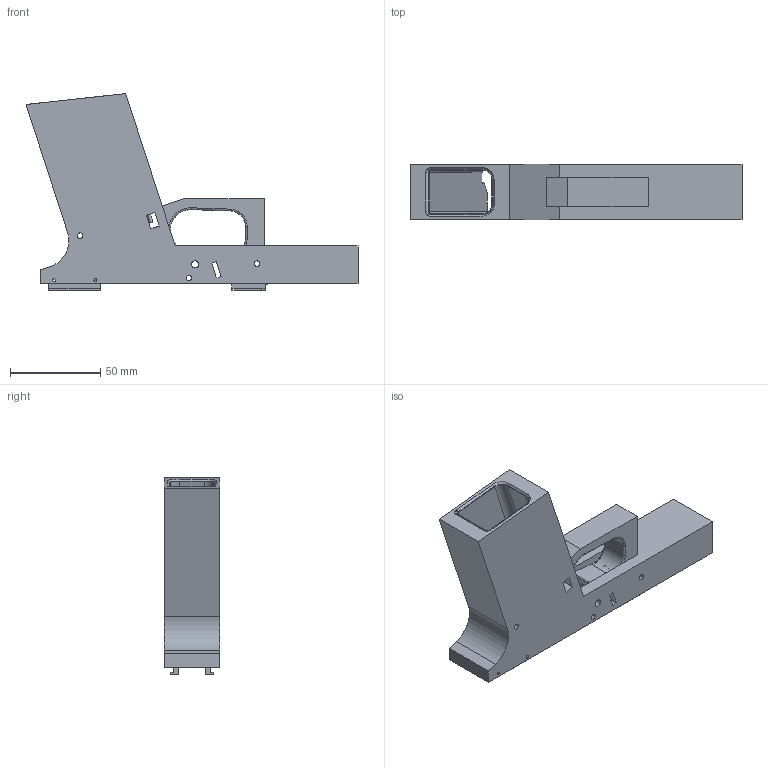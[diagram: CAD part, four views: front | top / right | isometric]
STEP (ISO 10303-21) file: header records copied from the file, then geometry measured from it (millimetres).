
FILE_DESCRIPTION(/* description */ (''),/* implementation_level */ '2;1');
FILE_NAME(/* name */ 'glock blank.stp',/* time_stamp */ '2019-10-25T14:33:53+03:00',/* author */ (''),/* organization */ (''),/* preprocessor_version */ 'ST-DEVELOPER v15.2',/* originating_system */ 'Autodesk Translator Framework v2.0.0.5431',/* authorisation */ '');
FILE_SCHEMA (('AUTOMOTIVE_DESIGN { 1 0 10303 214 3 1 1 }'));
Length unit declared in the file: centimetre
Products named in the file (1): GLOCK BLANK
Bounding box: 183.84 x 30.6 x 108.94 mm (x, y, z)
Volume: 141715.2 mm3; surface area: 57070.6 mm2
Topology: 5 solids, 5 shells, 683 faces, 1770 edges, 1057 vertices
Faces by surface type: cylinder 254, plane 199, bspline 121, torus 80, sphere 17, cone 12
Full cylindrical faces by diameter (mm): 1.655 x8, 1.8 x1, 3.057 x4, 3.06 x3, 4.042 x2
Entity records: 23574 total; most frequent: CARTESIAN_POINT 7395, ORIENTED_EDGE 3410, DIRECTION 3353, EDGE_CURVE 1705, AXIS2_PLACEMENT_3D 1282, VERTEX_POINT 1046, LINE 789, VECTOR 789
